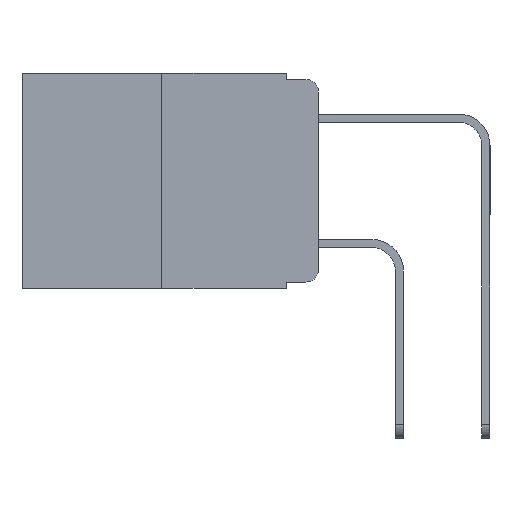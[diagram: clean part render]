
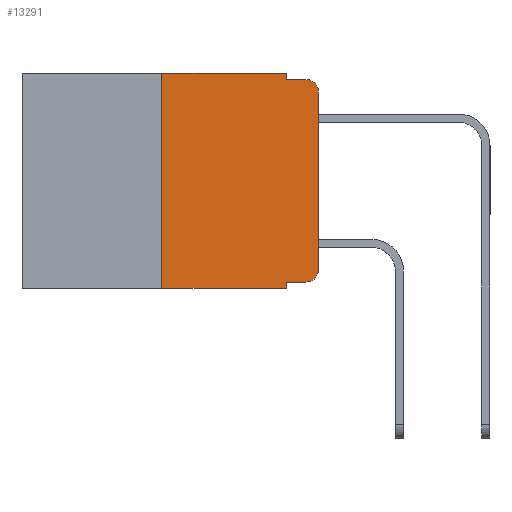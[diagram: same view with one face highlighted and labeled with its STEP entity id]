
A CAD part, left-side view. The second image highlights one B-rep face of the part: STEP entity #13291.
In plain terms, the highlighted planar face has unit normal (-1, 0, 0).
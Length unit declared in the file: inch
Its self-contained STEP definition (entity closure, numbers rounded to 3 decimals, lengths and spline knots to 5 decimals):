
#105 = CARTESIAN_POINT ( 'NONE',  ( 0., 0.473, 0. ) ) ;
#282 = EDGE_CURVE ( 'NONE', #14584, #12365, #508, .T. ) ;
#508 = LINE ( 'NONE', #8610, #14790 ) ;
#518 = LINE ( 'NONE', #16958, #11357 ) ;
#647 = ORIENTED_EDGE ( 'NONE', *, *, #16708, .F. ) ;
#751 = CARTESIAN_POINT ( 'NONE',  ( 0., 0.051, 0. ) ) ;
#940 = CARTESIAN_POINT ( 'NONE',  ( 0., 0.02, -0.313 ) ) ;
#1034 = VERTEX_POINT ( 'NONE', #13755 ) ;
#1158 = VERTEX_POINT ( 'NONE', #751 ) ;
#1193 = VERTEX_POINT ( 'NONE', #16068 ) ;
#1372 = VERTEX_POINT ( 'NONE', #11946 ) ;
#1391 = ORIENTED_EDGE ( 'NONE', *, *, #12881, .T. ) ;
#1998 = VERTEX_POINT ( 'NONE', #9656 ) ;
#2566 = VERTEX_POINT ( 'NONE', #17347 ) ;
#2574 = DIRECTION ( 'NONE',  ( 0., 0., -1. ) ) ;
#2780 = CIRCLE ( 'NONE', #15456, 0.02 ) ;
#2832 = DIRECTION ( 'NONE',  ( 0., 0., 1. ) ) ;
#2965 = DIRECTION ( 'NONE',  ( 0., -1., 0. ) ) ;
#3092 = LINE ( 'NONE', #14697, #10346 ) ;
#3298 = CARTESIAN_POINT ( 'NONE',  ( 0., 0.02, -0.01 ) ) ;
#3988 = EDGE_CURVE ( 'NONE', #1158, #14584, #5569, .T. ) ;
#4029 = PLANE ( 'NONE',  #17576 ) ;
#4385 = CARTESIAN_POINT ( 'NONE',  ( 0., 0.051, 0. ) ) ;
#4458 = CARTESIAN_POINT ( 'NONE',  ( 0., 0.051, -0.333 ) ) ;
#4808 = CARTESIAN_POINT ( 'NONE',  ( 0., 0.02, -0.333 ) ) ;
#4870 = DIRECTION ( 'NONE',  ( 0., -1., 0. ) ) ;
#5431 = DIRECTION ( 'NONE',  ( 0., 0., -1. ) ) ;
#5521 = DIRECTION ( 'NONE',  ( -1., 0., 0. ) ) ;
#5569 = LINE ( 'NONE', #4385, #15245 ) ;
#6358 = CARTESIAN_POINT ( 'NONE',  ( 0., 0.051, -0.333 ) ) ;
#6528 = ORIENTED_EDGE ( 'NONE', *, *, #12730, .T. ) ;
#6756 = CARTESIAN_POINT ( 'NONE',  ( 0., 0.473, 0. ) ) ;
#6781 = LINE ( 'NONE', #4458, #16765 ) ;
#6863 = VECTOR ( 'NONE', #2965, 39.37008 ) ;
#6952 = VECTOR ( 'NONE', #14060, 39.37008 ) ;
#6969 = EDGE_CURVE ( 'NONE', #1372, #1158, #10451, .T. ) ;
#7747 = ORIENTED_EDGE ( 'NONE', *, *, #6969, .F. ) ;
#8148 = ORIENTED_EDGE ( 'NONE', *, *, #12021, .T. ) ;
#8229 = VECTOR ( 'NONE', #2832, 39.37008 ) ;
#8476 = DIRECTION ( 'NONE',  ( 0., 0., -1. ) ) ;
#8610 = CARTESIAN_POINT ( 'NONE',  ( 0., 0.051, -0.01 ) ) ;
#9132 = CARTESIAN_POINT ( 'NONE',  ( 0., 0.051, -0.01 ) ) ;
#9656 = CARTESIAN_POINT ( 'NONE',  ( 0., 0., -0.03 ) ) ;
#10346 = VECTOR ( 'NONE', #15985, 39.37008 ) ;
#10451 = LINE ( 'NONE', #105, #6952 ) ;
#10612 = ORIENTED_EDGE ( 'NONE', *, *, #282, .F. ) ;
#10799 = DIRECTION ( 'NONE',  ( -1., 0., 0. ) ) ;
#10976 = CARTESIAN_POINT ( 'NONE',  ( 0., 0., 0. ) ) ;
#11357 = VECTOR ( 'NONE', #15743, 39.37008 ) ;
#11498 = ORIENTED_EDGE ( 'NONE', *, *, #13495, .T. ) ;
#11637 = VERTEX_POINT ( 'NONE', #4808 ) ;
#11946 = CARTESIAN_POINT ( 'NONE',  ( 0., 0.25, 0. ) ) ;
#12021 = EDGE_CURVE ( 'NONE', #1998, #12365, #2780, .T. ) ;
#12365 = VERTEX_POINT ( 'NONE', #3298 ) ;
#12453 = CARTESIAN_POINT ( 'NONE',  ( 0., 0.473, -0.343 ) ) ;
#12494 = ORIENTED_EDGE ( 'NONE', *, *, #15536, .F. ) ;
#12635 = EDGE_LOOP ( 'NONE', ( #1391, #8148, #10612, #16692, #7747, #647, #17286, #12494, #11498, #6528 ) ) ;
#12730 = EDGE_CURVE ( 'NONE', #11637, #2566, #13771, .T. ) ;
#12881 = EDGE_CURVE ( 'NONE', #2566, #1998, #15165, .T. ) ;
#13291 = ADVANCED_FACE ( 'NONE', ( #16580 ), #4029, .F. ) ;
#13372 = DIRECTION ( 'NONE',  ( 1., 0., 0. ) ) ;
#13454 = CARTESIAN_POINT ( 'NONE',  ( 0., 0.02, -0.03 ) ) ;
#13495 = EDGE_CURVE ( 'NONE', #14506, #11637, #6781, .T. ) ;
#13755 = CARTESIAN_POINT ( 'NONE',  ( 0., 0.051, -0.343 ) ) ;
#13771 = CIRCLE ( 'NONE', #17349, 0.02 ) ;
#14060 = DIRECTION ( 'NONE',  ( 0., -1., 0. ) ) ;
#14506 = VERTEX_POINT ( 'NONE', #6358 ) ;
#14584 = VERTEX_POINT ( 'NONE', #9132 ) ;
#14697 = CARTESIAN_POINT ( 'NONE',  ( 0., 0.051, 0. ) ) ;
#14743 = DIRECTION ( 'NONE',  ( 0., 0., -1. ) ) ;
#14790 = VECTOR ( 'NONE', #4870, 39.37008 ) ;
#15033 = EDGE_CURVE ( 'NONE', #1193, #1034, #17228, .T. ) ;
#15165 = LINE ( 'NONE', #10976, #8229 ) ;
#15245 = VECTOR ( 'NONE', #8476, 39.37008 ) ;
#15456 = AXIS2_PLACEMENT_3D ( 'NONE', #13454, #5521, #14743 ) ;
#15536 = EDGE_CURVE ( 'NONE', #14506, #1034, #3092, .T. ) ;
#15743 = DIRECTION ( 'NONE',  ( 0., 0., 1. ) ) ;
#15985 = DIRECTION ( 'NONE',  ( 0., 0., -1. ) ) ;
#16068 = CARTESIAN_POINT ( 'NONE',  ( 0., 0.25, -0.343 ) ) ;
#16271 = DIRECTION ( 'NONE',  ( 0., -1., 0. ) ) ;
#16580 = FACE_OUTER_BOUND ( 'NONE', #12635, .T. ) ;
#16692 = ORIENTED_EDGE ( 'NONE', *, *, #3988, .F. ) ;
#16708 = EDGE_CURVE ( 'NONE', #1193, #1372, #518, .T. ) ;
#16765 = VECTOR ( 'NONE', #16271, 39.37008 ) ;
#16958 = CARTESIAN_POINT ( 'NONE',  ( 0., 0.25, 0. ) ) ;
#17228 = LINE ( 'NONE', #12453, #6863 ) ;
#17286 = ORIENTED_EDGE ( 'NONE', *, *, #15033, .T. ) ;
#17347 = CARTESIAN_POINT ( 'NONE',  ( 0., 0., -0.313 ) ) ;
#17349 = AXIS2_PLACEMENT_3D ( 'NONE', #940, #10799, #2574 ) ;
#17576 = AXIS2_PLACEMENT_3D ( 'NONE', #6756, #13372, #5431 ) ;
